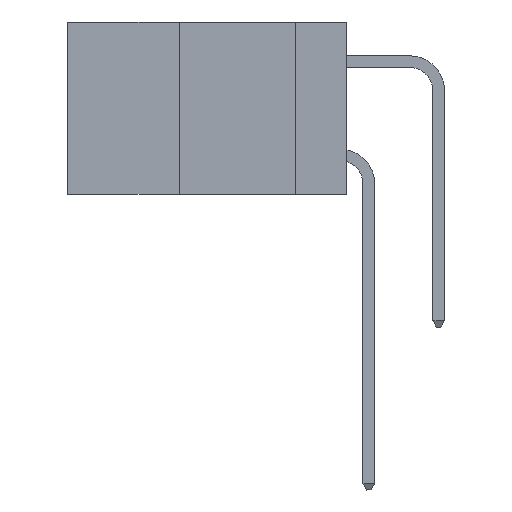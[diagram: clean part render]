
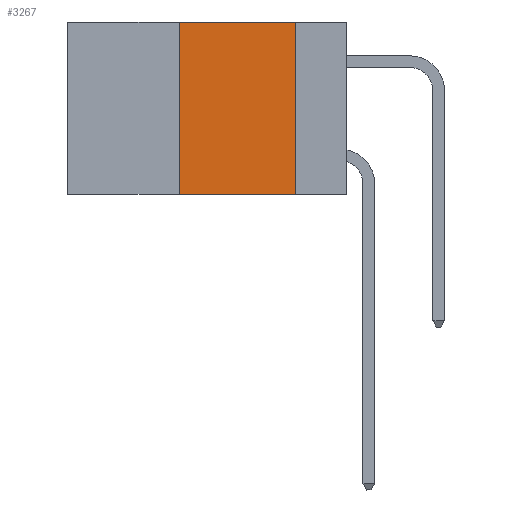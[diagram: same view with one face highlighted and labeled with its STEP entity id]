
A CAD part, left-side view. The second image highlights one B-rep face of the part: STEP entity #3267.
In plain terms, the highlighted planar face has unit normal (-1, 0, 0).
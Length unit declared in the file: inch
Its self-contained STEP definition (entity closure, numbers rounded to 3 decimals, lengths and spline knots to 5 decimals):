
#332 = VERTEX_POINT ( 'NONE', #10751 ) ;
#420 = CARTESIAN_POINT ( 'NONE',  ( 0., 0.6, 0. ) ) ;
#698 = VECTOR ( 'NONE', #3353, 39.37008 ) ;
#1215 = CARTESIAN_POINT ( 'NONE',  ( 0., 0.6, -0.37 ) ) ;
#1484 = EDGE_CURVE ( 'NONE', #332, #1900, #8028, .T. ) ;
#1787 = CARTESIAN_POINT ( 'NONE',  ( 0., 0.11, 0. ) ) ;
#1900 = VERTEX_POINT ( 'NONE', #5321 ) ;
#2553 = LINE ( 'NONE', #9590, #6722 ) ;
#2667 = VECTOR ( 'NONE', #4892, 39.37008 ) ;
#3267 = ADVANCED_FACE ( 'NONE', ( #12422 ), #6053, .F. ) ;
#3353 = DIRECTION ( 'NONE',  ( 0., 0., 1. ) ) ;
#4302 = ORIENTED_EDGE ( 'NONE', *, *, #13829, .F. ) ;
#4764 = DIRECTION ( 'NONE',  ( 1., 0., 0. ) ) ;
#4892 = DIRECTION ( 'NONE',  ( 0., -1., 0. ) ) ;
#5321 = CARTESIAN_POINT ( 'NONE',  ( 0., 0.11, -0.37 ) ) ;
#6053 = PLANE ( 'NONE',  #10208 ) ;
#6271 = DIRECTION ( 'NONE',  ( 0., -1., 0. ) ) ;
#6310 = VERTEX_POINT ( 'NONE', #1787 ) ;
#6622 = LINE ( 'NONE', #11748, #8047 ) ;
#6722 = VECTOR ( 'NONE', #6271, 39.37008 ) ;
#7110 = EDGE_CURVE ( 'NONE', #332, #7183, #10299, .T. ) ;
#7183 = VERTEX_POINT ( 'NONE', #10146 ) ;
#7756 = ORIENTED_EDGE ( 'NONE', *, *, #7110, .F. ) ;
#8028 = LINE ( 'NONE', #1215, #2667 ) ;
#8047 = VECTOR ( 'NONE', #11788, 39.37008 ) ;
#9412 = EDGE_CURVE ( 'NONE', #7183, #6310, #2553, .T. ) ;
#9590 = CARTESIAN_POINT ( 'NONE',  ( 0., 0.6, 0. ) ) ;
#10146 = CARTESIAN_POINT ( 'NONE',  ( 0., 0.36, 0. ) ) ;
#10208 = AXIS2_PLACEMENT_3D ( 'NONE', #420, #4764, #12679 ) ;
#10299 = LINE ( 'NONE', #11136, #698 ) ;
#10751 = CARTESIAN_POINT ( 'NONE',  ( 0., 0.36, -0.37 ) ) ;
#11136 = CARTESIAN_POINT ( 'NONE',  ( 0., 0.36, 0. ) ) ;
#11389 = ORIENTED_EDGE ( 'NONE', *, *, #9412, .F. ) ;
#11748 = CARTESIAN_POINT ( 'NONE',  ( 0., 0.11, 0. ) ) ;
#11788 = DIRECTION ( 'NONE',  ( 0., 0., -1. ) ) ;
#12422 = FACE_OUTER_BOUND ( 'NONE', #14373, .T. ) ;
#12679 = DIRECTION ( 'NONE',  ( 0., 0., -1. ) ) ;
#13777 = ORIENTED_EDGE ( 'NONE', *, *, #1484, .T. ) ;
#13829 = EDGE_CURVE ( 'NONE', #6310, #1900, #6622, .T. ) ;
#14373 = EDGE_LOOP ( 'NONE', ( #4302, #11389, #7756, #13777 ) ) ;
